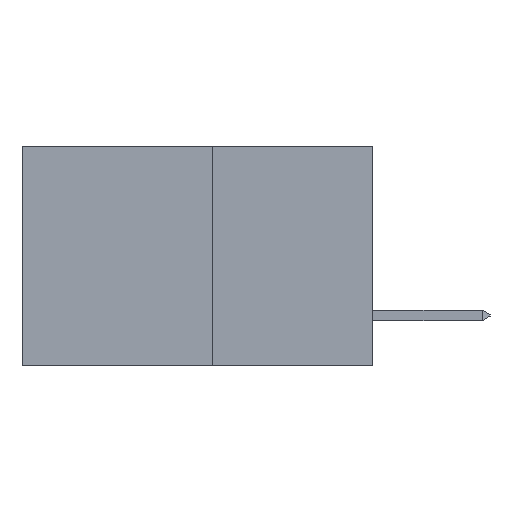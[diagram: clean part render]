
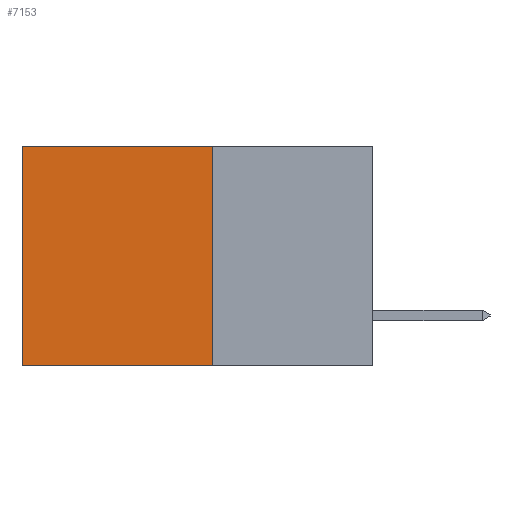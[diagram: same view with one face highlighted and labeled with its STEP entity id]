
A CAD part, left-side view. The second image highlights one B-rep face of the part: STEP entity #7153.
In plain terms, the highlighted planar face has unit normal (-1, 0, 0).
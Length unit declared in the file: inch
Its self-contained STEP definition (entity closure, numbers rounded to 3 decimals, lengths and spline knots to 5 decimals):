
#170 = VECTOR ( 'NONE', #1612, 39.37008 ) ;
#625 = EDGE_CURVE ( 'NONE', #9117, #2583, #2491, .T. ) ;
#661 = ORIENTED_EDGE ( 'NONE', *, *, #625, .T. ) ;
#796 = CARTESIAN_POINT ( 'NONE',  ( 0.277, 0.27, -0.37 ) ) ;
#1284 = CARTESIAN_POINT ( 'NONE',  ( 0.277, 0.27, 0. ) ) ;
#1612 = DIRECTION ( 'NONE',  ( 0., 1., 0. ) ) ;
#1789 = CARTESIAN_POINT ( 'NONE',  ( 0.277, 0.59, -0.37 ) ) ;
#2141 = CARTESIAN_POINT ( 'NONE',  ( 0.277, 0.27, -0.37 ) ) ;
#2171 = VECTOR ( 'NONE', #6259, 39.37008 ) ;
#2383 = ORIENTED_EDGE ( 'NONE', *, *, #8826, .F. ) ;
#2491 = LINE ( 'NONE', #1284, #2171 ) ;
#2583 = VERTEX_POINT ( 'NONE', #11217 ) ;
#2809 = DIRECTION ( 'NONE',  ( 0., 0., -1. ) ) ;
#2842 = LINE ( 'NONE', #6251, #170 ) ;
#3164 = DIRECTION ( 'NONE',  ( 1., 0., 0. ) ) ;
#3271 = ORIENTED_EDGE ( 'NONE', *, *, #11250, .T. ) ;
#4042 = EDGE_LOOP ( 'NONE', ( #3271, #6991, #2383, #661 ) ) ;
#4593 = VECTOR ( 'NONE', #2809, 39.37008 ) ;
#4613 = AXIS2_PLACEMENT_3D ( 'NONE', #2141, #3164, #12562 ) ;
#4906 = LINE ( 'NONE', #1789, #4593 ) ;
#6251 = CARTESIAN_POINT ( 'NONE',  ( 0.277, 0.27, -0.37 ) ) ;
#6259 = DIRECTION ( 'NONE',  ( 0., 1., 0. ) ) ;
#6379 = CARTESIAN_POINT ( 'NONE',  ( 0.277, 0.27, -0.37 ) ) ;
#6991 = ORIENTED_EDGE ( 'NONE', *, *, #7057, .F. ) ;
#7057 = EDGE_CURVE ( 'NONE', #7844, #7397, #2842, .T. ) ;
#7153 = ADVANCED_FACE ( 'NONE', ( #9143 ), #9304, .F. ) ;
#7397 = VERTEX_POINT ( 'NONE', #12301 ) ;
#7844 = VERTEX_POINT ( 'NONE', #6379 ) ;
#8748 = DIRECTION ( 'NONE',  ( 0., 0., -1. ) ) ;
#8826 = EDGE_CURVE ( 'NONE', #9117, #7844, #11810, .T. ) ;
#9117 = VERTEX_POINT ( 'NONE', #11982 ) ;
#9143 = FACE_OUTER_BOUND ( 'NONE', #4042, .T. ) ;
#9269 = VECTOR ( 'NONE', #8748, 39.37008 ) ;
#9304 = PLANE ( 'NONE',  #4613 ) ;
#11217 = CARTESIAN_POINT ( 'NONE',  ( 0.277, 0.59, 0. ) ) ;
#11250 = EDGE_CURVE ( 'NONE', #2583, #7397, #4906, .T. ) ;
#11810 = LINE ( 'NONE', #796, #9269 ) ;
#11982 = CARTESIAN_POINT ( 'NONE',  ( 0.277, 0.27, 0. ) ) ;
#12301 = CARTESIAN_POINT ( 'NONE',  ( 0.277, 0.59, -0.37 ) ) ;
#12562 = DIRECTION ( 'NONE',  ( 0., 0., -1. ) ) ;
